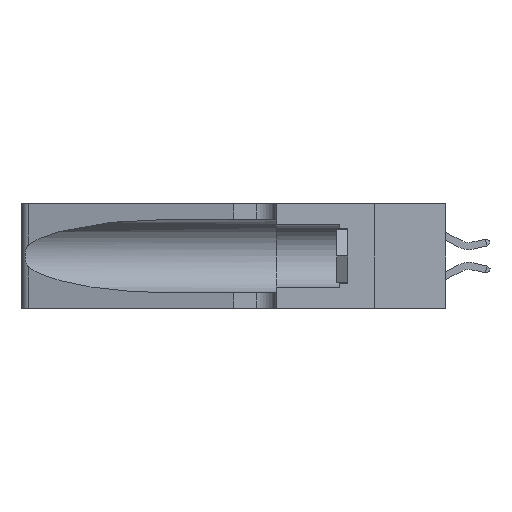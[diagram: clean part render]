
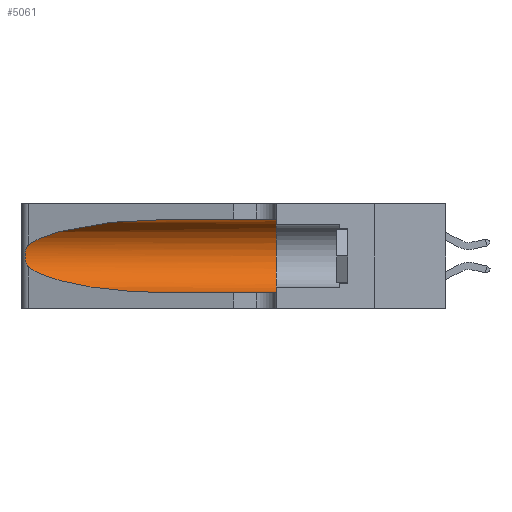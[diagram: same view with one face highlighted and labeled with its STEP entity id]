
A CAD part, left-side view. The second image highlights one B-rep face of the part: STEP entity #5061.
In plain terms, the highlighted cylindrical face has radius 3.308 mm (diameter 6.617 mm), a partial arc.
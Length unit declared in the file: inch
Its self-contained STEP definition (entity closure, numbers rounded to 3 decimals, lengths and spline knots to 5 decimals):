
#283 = CARTESIAN_POINT ( 'NONE',  ( 0.25487, 1.22718, 0.22369 ) ) ;
#726 = CARTESIAN_POINT ( 'NONE',  ( 0.18966, 0.96281, 0.31525 ) ) ;
#1312 = CARTESIAN_POINT ( 'NONE',  ( 0.25487, 1.22718, 0.22369 ) ) ;
#1548 = CARTESIAN_POINT ( 'NONE',  ( 0.1305, 0.35, 0.05475 ) ) ;
#1628 = VERTEX_POINT ( 'NONE', #283 ) ;
#1894 = EDGE_CURVE ( 'NONE', #1628, #13111, #16751, .T. ) ;
#2089 = CARTESIAN_POINT ( 'NONE',  ( 0.25555, 1.22994, 0.2215 ) ) ;
#2092 = CARTESIAN_POINT ( 'NONE',  ( 0.25856, 1.23593, 0.16098 ) ) ;
#2136 = CARTESIAN_POINT ( 'NONE',  ( 0.26075, 1.23896, 0.19203 ) ) ;
#2153 = CARTESIAN_POINT ( 'NONE',  ( 0.25787, 1.23484, 0.2124 ) ) ;
#2276 = CARTESIAN_POINT ( 'NONE',  ( 0.25487, 1.22718, 0.22369 ) ) ;
#2543 = DIRECTION ( 'NONE',  ( 0., -1., 0. ) ) ;
#2552 = DIRECTION ( 'NONE',  ( 0., -1., 0. ) ) ;
#2750 = CARTESIAN_POINT ( 'NONE',  ( 0.25639, 1.23184, 0.21858 ) ) ;
#2991 = CARTESIAN_POINT ( 'NONE',  ( 0.1305, 0.72297, 0.31525 ) ) ;
#3303 = ORIENTED_EDGE ( 'NONE', *, *, #13252, .F. ) ;
#3679 =( BOUNDED_CURVE ( )  B_SPLINE_CURVE ( 3, ( #16914, #726, #11176, #2276 ),
 .UNSPECIFIED., .F., .F. ) 
 B_SPLINE_CURVE_WITH_KNOTS ( ( 4, 4 ),
 ( 1.5708, 2.84003 ),
 .UNSPECIFIED. ) 
 CURVE ( )  GEOMETRIC_REPRESENTATION_ITEM ( )  RATIONAL_B_SPLINE_CURVE ( ( 1., 0.87, 0.87, 1. ) ) 
 REPRESENTATION_ITEM ( '' )  );
#3909 = CARTESIAN_POINT ( 'NONE',  ( 0.25854, 1.2359, 0.20912 ) ) ;
#3947 = CARTESIAN_POINT ( 'NONE',  ( 0.26018, 1.23835, 0.19895 ) ) ;
#4001 = CARTESIAN_POINT ( 'NONE',  ( 0.1305, 1.61858, 0.185 ) ) ;
#4159 = FACE_OUTER_BOUND ( 'NONE', #6738, .T. ) ;
#5061 = ADVANCED_FACE ( 'NONE', ( #4159 ), #11082, .F. ) ;
#5706 = EDGE_CURVE ( 'NONE', #16710, #12866, #15554, .T. ) ;
#5720 = ORIENTED_EDGE ( 'NONE', *, *, #1894, .T. ) ;
#6398 = CARTESIAN_POINT ( 'NONE',  ( 0.25487, 1.22718, 0.14631 ) ) ;
#6640 = ORIENTED_EDGE ( 'NONE', *, *, #10058, .T. ) ;
#6701 = CARTESIAN_POINT ( 'NONE',  ( 0.1305, 0.72297, 0.05475 ) ) ;
#6738 = EDGE_LOOP ( 'NONE', ( #7810, #5720, #6640, #13778, #18119, #3303 ) ) ;
#7810 = ORIENTED_EDGE ( 'NONE', *, *, #15817, .T. ) ;
#7899 = CARTESIAN_POINT ( 'NONE',  ( 0.1305, 0.35, 0.185 ) ) ;
#8519 = CARTESIAN_POINT ( 'NONE',  ( 0.1305, 1.61858, 0.31525 ) ) ;
#8656 = CARTESIAN_POINT ( 'NONE',  ( 0.1305, 0.72297, 0.05475 ) ) ;
#9058 = AXIS2_PLACEMENT_3D ( 'NONE', #4001, #2543, #12848 ) ;
#9425 = DIRECTION ( 'NONE',  ( 0., 0., 1. ) ) ;
#9571 = VECTOR ( 'NONE', #2552, 39.37008 ) ;
#10058 = EDGE_CURVE ( 'NONE', #13111, #14621, #17880, .T. ) ;
#10563 = DIRECTION ( 'NONE',  ( 0., -1., 0. ) ) ;
#11082 = CYLINDRICAL_SURFACE ( 'NONE', #9058, 0.13025 ) ;
#11176 = CARTESIAN_POINT ( 'NONE',  ( 0.2373, 1.15595, 0.28018 ) ) ;
#11498 = CARTESIAN_POINT ( 'NONE',  ( 0.2373, 1.15595, 0.08982 ) ) ;
#12159 = VERTEX_POINT ( 'NONE', #2991 ) ;
#12848 = DIRECTION ( 'NONE',  ( 0., 0., -1. ) ) ;
#12866 = VERTEX_POINT ( 'NONE', #1548 ) ;
#12896 = EDGE_CURVE ( 'NONE', #14621, #12866, #16781, .T. ) ;
#13111 = VERTEX_POINT ( 'NONE', #18328 ) ;
#13140 = CARTESIAN_POINT ( 'NONE',  ( 0.1305, 0.35, 0.31525 ) ) ;
#13252 = EDGE_CURVE ( 'NONE', #12159, #16710, #13349, .T. ) ;
#13349 = LINE ( 'NONE', #8519, #9571 ) ;
#13778 = ORIENTED_EDGE ( 'NONE', *, *, #12896, .T. ) ;
#14621 = VERTEX_POINT ( 'NONE', #6701 ) ;
#14836 = CARTESIAN_POINT ( 'NONE',  ( 0.1305, 1.61858, 0.05475 ) ) ;
#15554 = CIRCLE ( 'NONE', #17398, 0.13025 ) ;
#15817 = EDGE_CURVE ( 'NONE', #12159, #1628, #3679, .T. ) ;
#15818 = CARTESIAN_POINT ( 'NONE',  ( 0.25487, 1.22718, 0.14631 ) ) ;
#15843 = VECTOR ( 'NONE', #10563, 39.37008 ) ;
#16710 = VERTEX_POINT ( 'NONE', #13140 ) ;
#16718 = CARTESIAN_POINT ( 'NONE',  ( 0.26017, 1.23833, 0.17102 ) ) ;
#16744 = CARTESIAN_POINT ( 'NONE',  ( 0.26075, 1.23896, 0.178 ) ) ;
#16751 = B_SPLINE_CURVE_WITH_KNOTS ( 'NONE', 3,
 ( #1312, #2089, #2750, #2153, #3909, #3947, #2136, #16744, #16718, #2092, #16769, #16862, #16864, #6398 ),
 .UNSPECIFIED., .F., .F.,
 ( 4, 2, 2, 2, 2, 2, 4 ),
 ( 0., 0.00027, 0.00053, 0.00107, 0.0016, 0.00187, 0.00214 ),
 .UNSPECIFIED. ) ;
#16769 = CARTESIAN_POINT ( 'NONE',  ( 0.25789, 1.23486, 0.15765 ) ) ;
#16781 = LINE ( 'NONE', #14836, #15843 ) ;
#16862 = CARTESIAN_POINT ( 'NONE',  ( 0.25639, 1.23186, 0.15144 ) ) ;
#16864 = CARTESIAN_POINT ( 'NONE',  ( 0.25555, 1.22993, 0.14849 ) ) ;
#16914 = CARTESIAN_POINT ( 'NONE',  ( 0.1305, 0.72297, 0.31525 ) ) ;
#17320 = CARTESIAN_POINT ( 'NONE',  ( 0.18966, 0.96281, 0.05475 ) ) ;
#17398 = AXIS2_PLACEMENT_3D ( 'NONE', #7899, #18046, #9425 ) ;
#17880 =( BOUNDED_CURVE ( )  B_SPLINE_CURVE ( 3, ( #15818, #11498, #17320, #8656 ),
 .UNSPECIFIED., .F., .T. ) 
 B_SPLINE_CURVE_WITH_KNOTS ( ( 4, 4 ),
 ( 3.44316, 4.71239 ),
 .UNSPECIFIED. ) 
 CURVE ( )  GEOMETRIC_REPRESENTATION_ITEM ( )  RATIONAL_B_SPLINE_CURVE ( ( 1., 0.87, 0.87, 1. ) ) 
 REPRESENTATION_ITEM ( '' )  );
#18046 = DIRECTION ( 'NONE',  ( 0., 1., 0. ) ) ;
#18119 = ORIENTED_EDGE ( 'NONE', *, *, #5706, .F. ) ;
#18328 = CARTESIAN_POINT ( 'NONE',  ( 0.25487, 1.22718, 0.14631 ) ) ;
